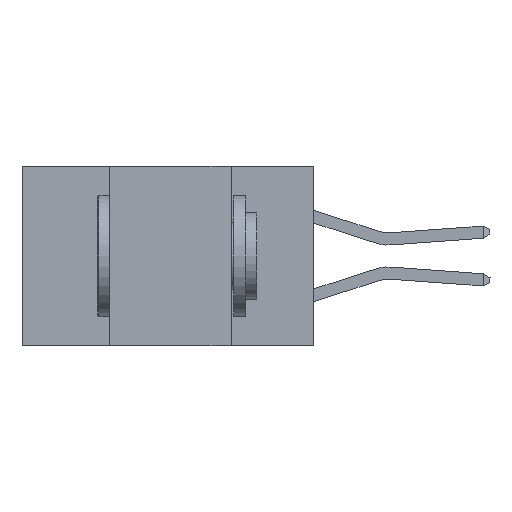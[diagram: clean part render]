
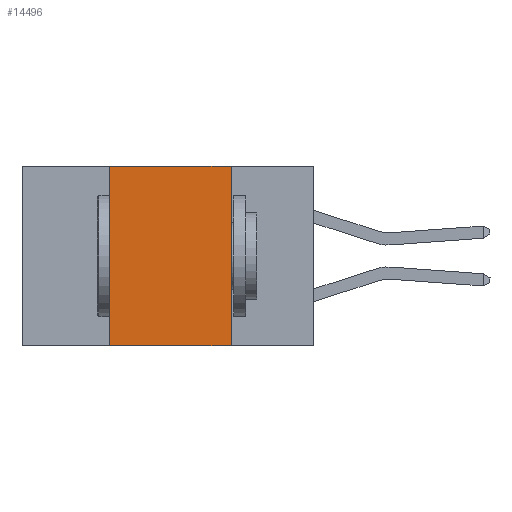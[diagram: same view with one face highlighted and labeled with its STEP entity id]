
A CAD part, left-side view. The second image highlights one B-rep face of the part: STEP entity #14496.
In plain terms, the highlighted planar face has unit normal (-1, 0, 0).
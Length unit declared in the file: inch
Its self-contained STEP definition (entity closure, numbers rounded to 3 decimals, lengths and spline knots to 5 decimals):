
#692 = VECTOR ( 'NONE', #4158, 39.37008 ) ;
#1135 = CARTESIAN_POINT ( 'NONE',  ( 0., 0.42, 0. ) ) ;
#1449 = LINE ( 'NONE', #13267, #692 ) ;
#2283 = LINE ( 'NONE', #10220, #8134 ) ;
#2912 = PLANE ( 'NONE',  #14348 ) ;
#3372 = CARTESIAN_POINT ( 'NONE',  ( 0., 0.6, 0. ) ) ;
#3395 = VERTEX_POINT ( 'NONE', #7004 ) ;
#4158 = DIRECTION ( 'NONE',  ( 0., 0., -1. ) ) ;
#4244 = EDGE_CURVE ( 'NONE', #12533, #6052, #2283, .T. ) ;
#4444 = ORIENTED_EDGE ( 'NONE', *, *, #9484, .F. ) ;
#4468 = ORIENTED_EDGE ( 'NONE', *, *, #5334, .F. ) ;
#4479 = ORIENTED_EDGE ( 'NONE', *, *, #4244, .F. ) ;
#4511 = ORIENTED_EDGE ( 'NONE', *, *, #7360, .T. ) ;
#5060 = CARTESIAN_POINT ( 'NONE',  ( 0., 0.17, -0.37 ) ) ;
#5334 = EDGE_CURVE ( 'NONE', #6052, #3395, #8638, .T. ) ;
#6035 = VECTOR ( 'NONE', #9362, 39.37008 ) ;
#6052 = VERTEX_POINT ( 'NONE', #1135 ) ;
#6431 = CARTESIAN_POINT ( 'NONE',  ( 0., 0.6, 0. ) ) ;
#7004 = CARTESIAN_POINT ( 'NONE',  ( 0., 0.17, 0. ) ) ;
#7360 = EDGE_CURVE ( 'NONE', #12533, #12289, #12101, .T. ) ;
#7600 = DIRECTION ( 'NONE',  ( 0., 0., -1. ) ) ;
#8134 = VECTOR ( 'NONE', #11458, 39.37008 ) ;
#8279 = VECTOR ( 'NONE', #12587, 39.37008 ) ;
#8638 = LINE ( 'NONE', #3372, #8279 ) ;
#9010 = EDGE_LOOP ( 'NONE', ( #4444, #4468, #4479, #4511 ) ) ;
#9362 = DIRECTION ( 'NONE',  ( 0., -1., 0. ) ) ;
#9484 = EDGE_CURVE ( 'NONE', #3395, #12289, #1449, .T. ) ;
#9692 = FACE_OUTER_BOUND ( 'NONE', #9010, .T. ) ;
#10220 = CARTESIAN_POINT ( 'NONE',  ( 0., 0.42, 0. ) ) ;
#11458 = DIRECTION ( 'NONE',  ( 0., 0., 1. ) ) ;
#11602 = CARTESIAN_POINT ( 'NONE',  ( 0., 0.6, -0.37 ) ) ;
#12101 = LINE ( 'NONE', #11602, #6035 ) ;
#12289 = VERTEX_POINT ( 'NONE', #5060 ) ;
#12533 = VERTEX_POINT ( 'NONE', #14630 ) ;
#12587 = DIRECTION ( 'NONE',  ( 0., -1., 0. ) ) ;
#13267 = CARTESIAN_POINT ( 'NONE',  ( 0., 0.17, 0. ) ) ;
#14348 = AXIS2_PLACEMENT_3D ( 'NONE', #6431, #14386, #7600 ) ;
#14386 = DIRECTION ( 'NONE',  ( 1., 0., 0. ) ) ;
#14496 = ADVANCED_FACE ( 'NONE', ( #9692 ), #2912, .F. ) ;
#14630 = CARTESIAN_POINT ( 'NONE',  ( 0., 0.42, -0.37 ) ) ;
